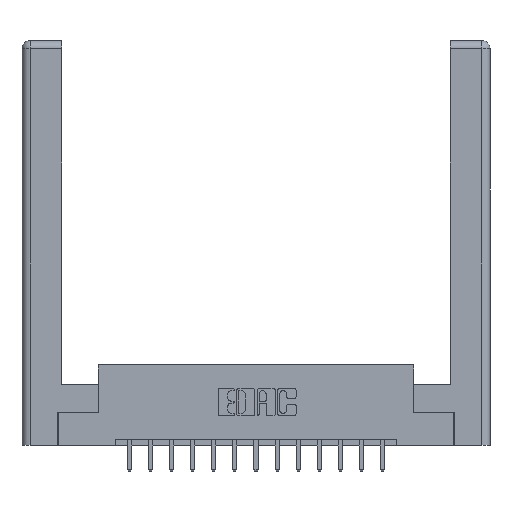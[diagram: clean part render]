
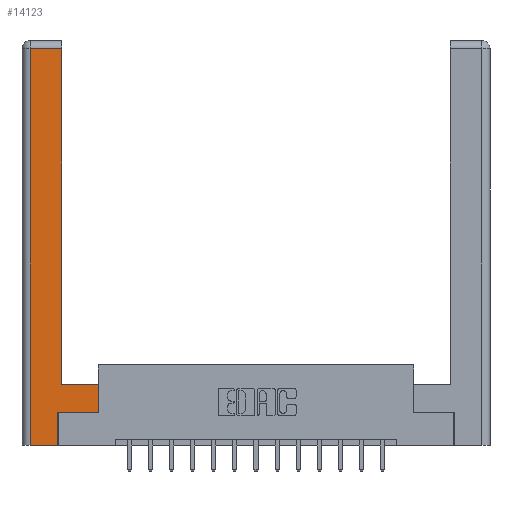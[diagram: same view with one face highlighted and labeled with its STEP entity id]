
A CAD part, top view. The second image highlights one B-rep face of the part: STEP entity #14123.
In plain terms, the highlighted planar face has unit normal (0, 0, 1).
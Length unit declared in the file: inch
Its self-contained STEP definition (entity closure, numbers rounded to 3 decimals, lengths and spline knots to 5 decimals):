
#271 = CARTESIAN_POINT ( 'NONE',  ( 0.295, 0.45, 0. ) ) ;
#510 = FACE_OUTER_BOUND ( 'NONE', #11317, .T. ) ;
#562 = ORIENTED_EDGE ( 'NONE', *, *, #7724, .T. ) ;
#806 = LINE ( 'NONE', #5105, #8217 ) ;
#835 = ORIENTED_EDGE ( 'NONE', *, *, #13044, .T. ) ;
#1315 = DIRECTION ( 'NONE',  ( -1., 0., 0. ) ) ;
#2193 = VERTEX_POINT ( 'NONE', #12979 ) ;
#2416 = DIRECTION ( 'NONE',  ( 0., -1., 0. ) ) ;
#2594 = CARTESIAN_POINT ( 'NONE',  ( 0.295, 3., 0. ) ) ;
#2636 = EDGE_CURVE ( 'NONE', #9379, #2714, #3249, .T. ) ;
#2645 = DIRECTION ( 'NONE',  ( 0., 1., 0. ) ) ;
#2706 = DIRECTION ( 'NONE',  ( 0., 1., 0. ) ) ;
#2714 = VERTEX_POINT ( 'NONE', #14466 ) ;
#2873 = CARTESIAN_POINT ( 'NONE',  ( 0.265, 0., 0. ) ) ;
#2884 = EDGE_CURVE ( 'NONE', #2714, #16546, #4842, .T. ) ;
#3249 = LINE ( 'NONE', #2873, #8830 ) ;
#3268 = EDGE_CURVE ( 'NONE', #13795, #9379, #806, .T. ) ;
#3398 = CARTESIAN_POINT ( 'NONE',  ( 0.265, 0.245, 0. ) ) ;
#3404 = AXIS2_PLACEMENT_3D ( 'NONE', #10493, #11782, #4102 ) ;
#3449 = LINE ( 'NONE', #7555, #5286 ) ;
#3505 = ORIENTED_EDGE ( 'NONE', *, *, #3268, .T. ) ;
#3519 = LINE ( 'NONE', #2594, #14335 ) ;
#4102 = DIRECTION ( 'NONE',  ( -1., 0., 0. ) ) ;
#4285 = LINE ( 'NONE', #271, #9072 ) ;
#4508 = CARTESIAN_POINT ( 'NONE',  ( 0.565, 0.45, 0. ) ) ;
#4842 = LINE ( 'NONE', #3398, #16428 ) ;
#5105 = CARTESIAN_POINT ( 'NONE',  ( 0.0615, 0., 0. ) ) ;
#5286 = VECTOR ( 'NONE', #1315, 39.37008 ) ;
#6129 = CARTESIAN_POINT ( 'NONE',  ( 0.565, 0.245, 0. ) ) ;
#6133 = VECTOR ( 'NONE', #12121, 39.37008 ) ;
#6529 = ORIENTED_EDGE ( 'NONE', *, *, #13589, .T. ) ;
#7017 = VERTEX_POINT ( 'NONE', #6129 ) ;
#7199 = EDGE_CURVE ( 'NONE', #16142, #2193, #4285, .T. ) ;
#7555 = CARTESIAN_POINT ( 'NONE',  ( 0.0615, 2.94, 0. ) ) ;
#7702 = VECTOR ( 'NONE', #2645, 39.37008 ) ;
#7724 = EDGE_CURVE ( 'NONE', #15515, #13795, #3449, .T. ) ;
#8217 = VECTOR ( 'NONE', #2416, 39.37008 ) ;
#8340 = DIRECTION ( 'NONE',  ( 1., 0., 0. ) ) ;
#8830 = VECTOR ( 'NONE', #8340, 39.37008 ) ;
#8882 = CARTESIAN_POINT ( 'NONE',  ( 0.565, 0.45, 0. ) ) ;
#9072 = VECTOR ( 'NONE', #9225, 39.37008 ) ;
#9225 = DIRECTION ( 'NONE',  ( -1., 0., 0. ) ) ;
#9379 = VERTEX_POINT ( 'NONE', #9524 ) ;
#9391 = ORIENTED_EDGE ( 'NONE', *, *, #2636, .T. ) ;
#9484 = LINE ( 'NONE', #10841, #6133 ) ;
#9524 = CARTESIAN_POINT ( 'NONE',  ( 0.0615, 0., 0. ) ) ;
#9926 = CARTESIAN_POINT ( 'NONE',  ( 0.0615, 2.94, 0. ) ) ;
#10286 = LINE ( 'NONE', #8882, #7702 ) ;
#10493 = CARTESIAN_POINT ( 'NONE',  ( 0., 0., 0. ) ) ;
#10567 = ORIENTED_EDGE ( 'NONE', *, *, #7199, .T. ) ;
#10841 = CARTESIAN_POINT ( 'NONE',  ( 0.565, 0.245, 0. ) ) ;
#11317 = EDGE_LOOP ( 'NONE', ( #835, #562, #3505, #9391, #13501, #6529, #14509, #10567 ) ) ;
#11782 = DIRECTION ( 'NONE',  ( 0., 0., -1. ) ) ;
#12053 = CARTESIAN_POINT ( 'NONE',  ( 0.295, 2.94, 0. ) ) ;
#12121 = DIRECTION ( 'NONE',  ( 1., 0., 0. ) ) ;
#12979 = CARTESIAN_POINT ( 'NONE',  ( 0.295, 0.45, 0. ) ) ;
#13044 = EDGE_CURVE ( 'NONE', #2193, #15515, #3519, .T. ) ;
#13501 = ORIENTED_EDGE ( 'NONE', *, *, #2884, .T. ) ;
#13589 = EDGE_CURVE ( 'NONE', #16546, #7017, #9484, .T. ) ;
#13795 = VERTEX_POINT ( 'NONE', #9926 ) ;
#14123 = ADVANCED_FACE ( 'NONE', ( #510 ), #15652, .F. ) ;
#14335 = VECTOR ( 'NONE', #2706, 39.37008 ) ;
#14466 = CARTESIAN_POINT ( 'NONE',  ( 0.265, 0., 0. ) ) ;
#14509 = ORIENTED_EDGE ( 'NONE', *, *, #15323, .T. ) ;
#15323 = EDGE_CURVE ( 'NONE', #7017, #16142, #10286, .T. ) ;
#15515 = VERTEX_POINT ( 'NONE', #12053 ) ;
#15652 = PLANE ( 'NONE',  #3404 ) ;
#16142 = VERTEX_POINT ( 'NONE', #4508 ) ;
#16241 = DIRECTION ( 'NONE',  ( 0., 1., 0. ) ) ;
#16315 = CARTESIAN_POINT ( 'NONE',  ( 0.265, 0.245, 0. ) ) ;
#16428 = VECTOR ( 'NONE', #16241, 39.37008 ) ;
#16546 = VERTEX_POINT ( 'NONE', #16315 ) ;
